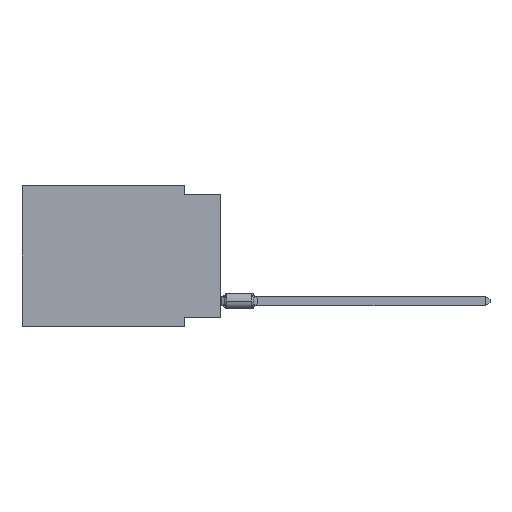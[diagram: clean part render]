
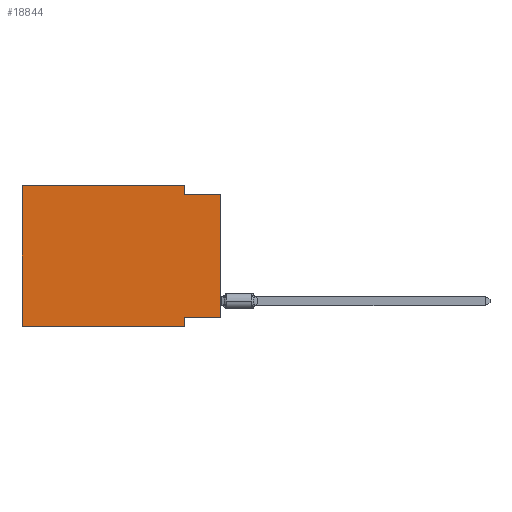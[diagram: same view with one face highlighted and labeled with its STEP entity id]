
A CAD part, left-side view. The second image highlights one B-rep face of the part: STEP entity #18844.
In plain terms, the highlighted planar face has unit normal (-1, 0, 0).
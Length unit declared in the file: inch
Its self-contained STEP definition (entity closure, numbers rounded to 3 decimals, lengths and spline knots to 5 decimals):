
#221 = EDGE_CURVE ( 'NONE', #9854, #64947, #56139, .T. ) ;
#1197 = VECTOR ( 'NONE', #80799, 39.37008 ) ;
#1559 = AXIS2_PLACEMENT_3D ( 'NONE', #10792, #9564, #54303 ) ;
#4144 = PLANE ( 'NONE',  #1559 ) ;
#4642 = DIRECTION ( 'NONE',  ( 0., 0., 1. ) ) ;
#5323 = VECTOR ( 'NONE', #68682, 39.37008 ) ;
#6086 = VERTEX_POINT ( 'NONE', #20488 ) ;
#7938 = VERTEX_POINT ( 'NONE', #75632 ) ;
#9564 = DIRECTION ( 'NONE',  ( 1., 0., 0. ) ) ;
#9705 = ORIENTED_EDGE ( 'NONE', *, *, #13423, .F. ) ;
#9762 = CARTESIAN_POINT ( 'NONE',  ( 0., 0.1, 0. ) ) ;
#9854 = VERTEX_POINT ( 'NONE', #16127 ) ;
#10792 = CARTESIAN_POINT ( 'NONE',  ( 0., 0.55, 0. ) ) ;
#10959 = VECTOR ( 'NONE', #30166, 39.37008 ) ;
#13407 = CARTESIAN_POINT ( 'NONE',  ( 0., 0.1, -0.39 ) ) ;
#13423 = EDGE_CURVE ( 'NONE', #39899, #7938, #25744, .T. ) ;
#13560 = DIRECTION ( 'NONE',  ( 0., 1., 0. ) ) ;
#16127 = CARTESIAN_POINT ( 'NONE',  ( 0., 0.1, -0.025 ) ) ;
#18844 = ADVANCED_FACE ( 'NONE', ( #66859 ), #4144, .F. ) ;
#19588 = VERTEX_POINT ( 'NONE', #48092 ) ;
#19959 = ORIENTED_EDGE ( 'NONE', *, *, #221, .F. ) ;
#20488 = CARTESIAN_POINT ( 'NONE',  ( 0., 0.55, -0.39 ) ) ;
#21124 = ORIENTED_EDGE ( 'NONE', *, *, #71374, .F. ) ;
#24999 = EDGE_LOOP ( 'NONE', ( #39172, #19959, #63697, #9705, #75975, #30635, #21124, #82099 ) ) ;
#25744 = LINE ( 'NONE', #51264, #75918 ) ;
#27320 = VECTOR ( 'NONE', #13560, 39.37008 ) ;
#29689 = DIRECTION ( 'NONE',  ( 0., 0., 1. ) ) ;
#29758 = LINE ( 'NONE', #69061, #10959 ) ;
#29893 = CARTESIAN_POINT ( 'NONE',  ( 0., 0., -0.365 ) ) ;
#30166 = DIRECTION ( 'NONE',  ( 0., -1., 0. ) ) ;
#30635 = ORIENTED_EDGE ( 'NONE', *, *, #47278, .T. ) ;
#32244 = CARTESIAN_POINT ( 'NONE',  ( 0., 0.55, 0. ) ) ;
#32580 = VERTEX_POINT ( 'NONE', #77405 ) ;
#33943 = EDGE_CURVE ( 'NONE', #6086, #39899, #36374, .T. ) ;
#34415 = LINE ( 'NONE', #9762, #1197 ) ;
#36374 = LINE ( 'NONE', #62734, #55154 ) ;
#38883 = DIRECTION ( 'NONE',  ( 0., 0., -1. ) ) ;
#39172 = ORIENTED_EDGE ( 'NONE', *, *, #41383, .T. ) ;
#39899 = VERTEX_POINT ( 'NONE', #32244 ) ;
#41383 = EDGE_CURVE ( 'NONE', #44121, #64947, #42238, .T. ) ;
#42238 = LINE ( 'NONE', #48522, #55797 ) ;
#44121 = VERTEX_POINT ( 'NONE', #29893 ) ;
#44477 = EDGE_CURVE ( 'NONE', #7938, #9854, #34415, .T. ) ;
#45326 = CARTESIAN_POINT ( 'NONE',  ( 0., 0., -0.365 ) ) ;
#47278 = EDGE_CURVE ( 'NONE', #6086, #19588, #29758, .T. ) ;
#48092 = CARTESIAN_POINT ( 'NONE',  ( 0., 0.1, -0.39 ) ) ;
#48522 = CARTESIAN_POINT ( 'NONE',  ( 0., 0., 0. ) ) ;
#51264 = CARTESIAN_POINT ( 'NONE',  ( 0., 0.55, 0. ) ) ;
#54303 = DIRECTION ( 'NONE',  ( 0., 0., -1. ) ) ;
#55154 = VECTOR ( 'NONE', #4642, 39.37008 ) ;
#55797 = VECTOR ( 'NONE', #29689, 39.37008 ) ;
#56139 = LINE ( 'NONE', #61603, #5323 ) ;
#61603 = CARTESIAN_POINT ( 'NONE',  ( 0., 0., -0.025 ) ) ;
#62734 = CARTESIAN_POINT ( 'NONE',  ( 0., 0.55, 0. ) ) ;
#63697 = ORIENTED_EDGE ( 'NONE', *, *, #44477, .F. ) ;
#64947 = VERTEX_POINT ( 'NONE', #82606 ) ;
#65048 = VECTOR ( 'NONE', #38883, 39.37008 ) ;
#66859 = FACE_OUTER_BOUND ( 'NONE', #24999, .T. ) ;
#68682 = DIRECTION ( 'NONE',  ( 0., -1., 0. ) ) ;
#69061 = CARTESIAN_POINT ( 'NONE',  ( 0., 0.55, -0.39 ) ) ;
#70014 = LINE ( 'NONE', #45326, #27320 ) ;
#71374 = EDGE_CURVE ( 'NONE', #32580, #19588, #76527, .T. ) ;
#75632 = CARTESIAN_POINT ( 'NONE',  ( 0., 0.1, 0. ) ) ;
#75918 = VECTOR ( 'NONE', #76745, 39.37008 ) ;
#75975 = ORIENTED_EDGE ( 'NONE', *, *, #33943, .F. ) ;
#76527 = LINE ( 'NONE', #13407, #65048 ) ;
#76745 = DIRECTION ( 'NONE',  ( 0., -1., 0. ) ) ;
#77405 = CARTESIAN_POINT ( 'NONE',  ( 0., 0.1, -0.365 ) ) ;
#80799 = DIRECTION ( 'NONE',  ( 0., 0., -1. ) ) ;
#81265 = EDGE_CURVE ( 'NONE', #44121, #32580, #70014, .T. ) ;
#82099 = ORIENTED_EDGE ( 'NONE', *, *, #81265, .F. ) ;
#82606 = CARTESIAN_POINT ( 'NONE',  ( 0., 0., -0.025 ) ) ;
